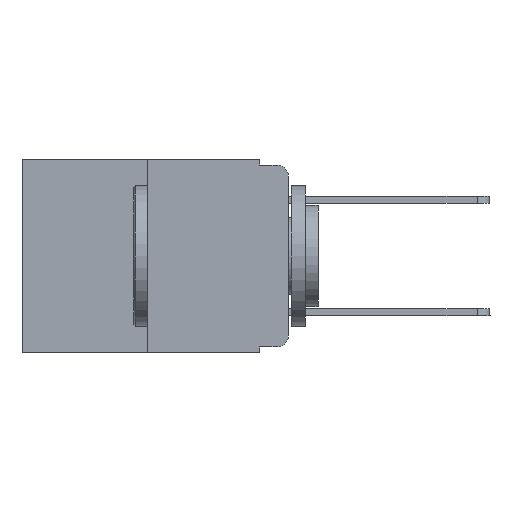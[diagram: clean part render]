
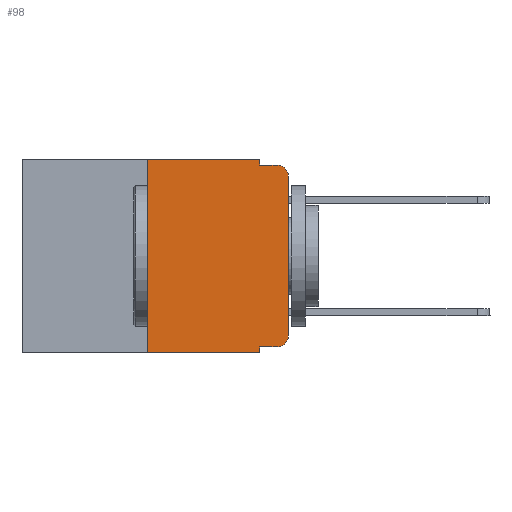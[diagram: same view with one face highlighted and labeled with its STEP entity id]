
A CAD part, left-side view. The second image highlights one B-rep face of the part: STEP entity #98.
In plain terms, the highlighted planar face has unit normal (-1, 0, 0).
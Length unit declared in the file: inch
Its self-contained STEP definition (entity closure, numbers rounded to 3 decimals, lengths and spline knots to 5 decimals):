
#98 = ADVANCED_FACE ( 'NONE', ( #2115 ), #9662, .F. ) ;
#343 = DIRECTION ( 'NONE',  ( 0., -1., 0. ) ) ;
#976 = DIRECTION ( 'NONE',  ( 0., 0., 1. ) ) ;
#1028 = AXIS2_PLACEMENT_3D ( 'NONE', #1947, #13858, #9839 ) ;
#1156 = ORIENTED_EDGE ( 'NONE', *, *, #14366, .T. ) ;
#1867 = DIRECTION ( 'NONE',  ( -1., 0., 0. ) ) ;
#1947 = CARTESIAN_POINT ( 'NONE',  ( 0., 0.473, 0. ) ) ;
#2115 = FACE_OUTER_BOUND ( 'NONE', #15448, .T. ) ;
#2213 = CARTESIAN_POINT ( 'NONE',  ( 0., 0.473, -0.343 ) ) ;
#2425 = LINE ( 'NONE', #2507, #6232 ) ;
#2507 = CARTESIAN_POINT ( 'NONE',  ( 0., 0.051, 0. ) ) ;
#2551 = DIRECTION ( 'NONE',  ( 0., 0., 1. ) ) ;
#2648 = VECTOR ( 'NONE', #343, 39.37008 ) ;
#2676 = EDGE_CURVE ( 'NONE', #6306, #3673, #5399, .T. ) ;
#2795 = VERTEX_POINT ( 'NONE', #12280 ) ;
#3020 = CIRCLE ( 'NONE', #16420, 0.02 ) ;
#3562 = ORIENTED_EDGE ( 'NONE', *, *, #12750, .F. ) ;
#3587 = VERTEX_POINT ( 'NONE', #12562 ) ;
#3644 = CARTESIAN_POINT ( 'NONE',  ( 0., 0.25, 0. ) ) ;
#3663 = ORIENTED_EDGE ( 'NONE', *, *, #6575, .F. ) ;
#3673 = VERTEX_POINT ( 'NONE', #12394 ) ;
#4153 = EDGE_CURVE ( 'NONE', #14869, #3587, #14035, .T. ) ;
#4201 = CARTESIAN_POINT ( 'NONE',  ( 0., 0.051, -0.333 ) ) ;
#5102 = EDGE_CURVE ( 'NONE', #16683, #3673, #5905, .T. ) ;
#5120 = LINE ( 'NONE', #14044, #9527 ) ;
#5130 = DIRECTION ( 'NONE',  ( -1., 0., 0. ) ) ;
#5233 = DIRECTION ( 'NONE',  ( 0., -1., 0. ) ) ;
#5257 = CARTESIAN_POINT ( 'NONE',  ( 0., 0., 0. ) ) ;
#5399 = LINE ( 'NONE', #11759, #10271 ) ;
#5697 = LINE ( 'NONE', #16423, #14226 ) ;
#5753 = CARTESIAN_POINT ( 'NONE',  ( 0., 0.051, -0.333 ) ) ;
#5819 = CARTESIAN_POINT ( 'NONE',  ( 0., 0., -0.03 ) ) ;
#5905 = CIRCLE ( 'NONE', #9471, 0.02 ) ;
#6232 = VECTOR ( 'NONE', #13144, 39.37008 ) ;
#6306 = VERTEX_POINT ( 'NONE', #15339 ) ;
#6467 = EDGE_CURVE ( 'NONE', #7742, #16541, #10630, .T. ) ;
#6503 = CARTESIAN_POINT ( 'NONE',  ( 0., 0.02, -0.333 ) ) ;
#6575 = EDGE_CURVE ( 'NONE', #7184, #2795, #14821, .T. ) ;
#6667 = CARTESIAN_POINT ( 'NONE',  ( 0., 0.02, -0.03 ) ) ;
#7025 = VECTOR ( 'NONE', #9862, 39.37008 ) ;
#7184 = VERTEX_POINT ( 'NONE', #3644 ) ;
#7500 = DIRECTION ( 'NONE',  ( 0., -1., 0. ) ) ;
#7579 = EDGE_CURVE ( 'NONE', #2795, #6306, #2425, .T. ) ;
#7742 = VERTEX_POINT ( 'NONE', #5753 ) ;
#8379 = DIRECTION ( 'NONE',  ( 0., 0., -1. ) ) ;
#8536 = ORIENTED_EDGE ( 'NONE', *, *, #7579, .F. ) ;
#9471 = AXIS2_PLACEMENT_3D ( 'NONE', #6667, #5130, #14480 ) ;
#9527 = VECTOR ( 'NONE', #2551, 39.37008 ) ;
#9662 = PLANE ( 'NONE',  #1028 ) ;
#9839 = DIRECTION ( 'NONE',  ( 0., 0., -1. ) ) ;
#9844 = VERTEX_POINT ( 'NONE', #15591 ) ;
#9862 = DIRECTION ( 'NONE',  ( 0., -1., 0. ) ) ;
#9942 = CARTESIAN_POINT ( 'NONE',  ( 0., 0.473, 0. ) ) ;
#10271 = VECTOR ( 'NONE', #5233, 39.37008 ) ;
#10518 = ORIENTED_EDGE ( 'NONE', *, *, #4153, .T. ) ;
#10630 = LINE ( 'NONE', #4201, #2648 ) ;
#11021 = CARTESIAN_POINT ( 'NONE',  ( 0., 0.25, -0.343 ) ) ;
#11161 = ORIENTED_EDGE ( 'NONE', *, *, #5102, .T. ) ;
#11759 = CARTESIAN_POINT ( 'NONE',  ( 0., 0.051, -0.01 ) ) ;
#12280 = CARTESIAN_POINT ( 'NONE',  ( 0., 0.051, 0. ) ) ;
#12328 = DIRECTION ( 'NONE',  ( 0., 0., -1. ) ) ;
#12394 = CARTESIAN_POINT ( 'NONE',  ( 0., 0.02, -0.01 ) ) ;
#12562 = CARTESIAN_POINT ( 'NONE',  ( 0., 0.051, -0.343 ) ) ;
#12601 = CARTESIAN_POINT ( 'NONE',  ( 0., 0.02, -0.313 ) ) ;
#12732 = VECTOR ( 'NONE', #7500, 39.37008 ) ;
#12750 = EDGE_CURVE ( 'NONE', #14869, #7184, #5120, .T. ) ;
#13144 = DIRECTION ( 'NONE',  ( 0., 0., -1. ) ) ;
#13858 = DIRECTION ( 'NONE',  ( 1., 0., 0. ) ) ;
#14014 = LINE ( 'NONE', #5257, #16190 ) ;
#14035 = LINE ( 'NONE', #2213, #12732 ) ;
#14044 = CARTESIAN_POINT ( 'NONE',  ( 0., 0.25, 0. ) ) ;
#14060 = ORIENTED_EDGE ( 'NONE', *, *, #14849, .F. ) ;
#14226 = VECTOR ( 'NONE', #12328, 39.37008 ) ;
#14348 = ORIENTED_EDGE ( 'NONE', *, *, #16197, .T. ) ;
#14366 = EDGE_CURVE ( 'NONE', #16541, #9844, #3020, .T. ) ;
#14480 = DIRECTION ( 'NONE',  ( 0., 0., -1. ) ) ;
#14750 = ORIENTED_EDGE ( 'NONE', *, *, #2676, .F. ) ;
#14821 = LINE ( 'NONE', #9942, #7025 ) ;
#14849 = EDGE_CURVE ( 'NONE', #7742, #3587, #5697, .T. ) ;
#14869 = VERTEX_POINT ( 'NONE', #11021 ) ;
#14881 = ORIENTED_EDGE ( 'NONE', *, *, #6467, .T. ) ;
#15339 = CARTESIAN_POINT ( 'NONE',  ( 0., 0.051, -0.01 ) ) ;
#15448 = EDGE_LOOP ( 'NONE', ( #14348, #11161, #14750, #8536, #3663, #3562, #10518, #14060, #14881, #1156 ) ) ;
#15591 = CARTESIAN_POINT ( 'NONE',  ( 0., 0., -0.313 ) ) ;
#16190 = VECTOR ( 'NONE', #976, 39.37008 ) ;
#16197 = EDGE_CURVE ( 'NONE', #9844, #16683, #14014, .T. ) ;
#16420 = AXIS2_PLACEMENT_3D ( 'NONE', #12601, #1867, #8379 ) ;
#16423 = CARTESIAN_POINT ( 'NONE',  ( 0., 0.051, 0. ) ) ;
#16541 = VERTEX_POINT ( 'NONE', #6503 ) ;
#16683 = VERTEX_POINT ( 'NONE', #5819 ) ;
